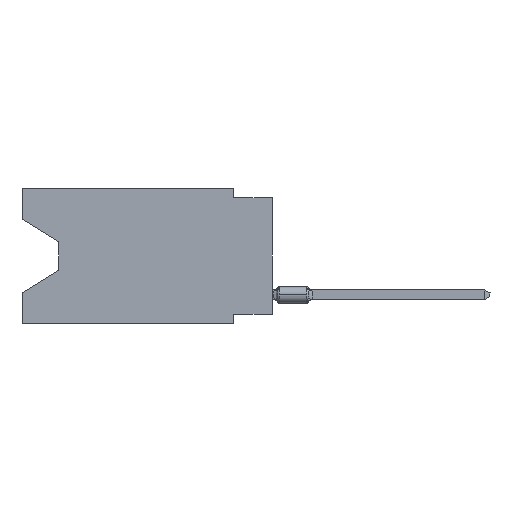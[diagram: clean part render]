
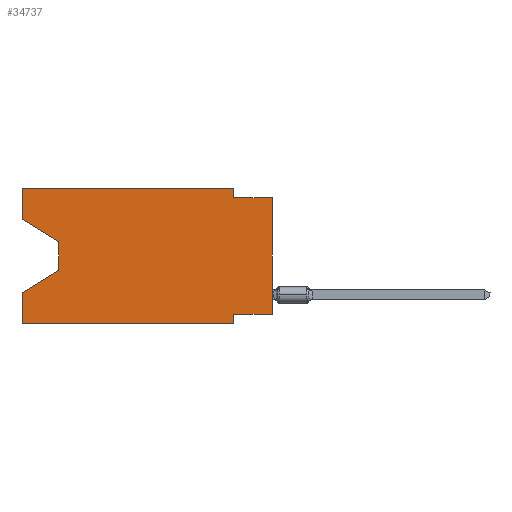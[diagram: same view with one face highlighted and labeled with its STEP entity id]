
A CAD part, left-side view. The second image highlights one B-rep face of the part: STEP entity #34737.
In plain terms, the highlighted planar face has unit normal (-1, 0, 0).
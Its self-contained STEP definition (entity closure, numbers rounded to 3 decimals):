
#1907 = EDGE_CURVE ( 'NONE', #35857, #26477, #60398, .T. ) ;
#2072 = CARTESIAN_POINT ( 'NONE',  ( 0., 16.383, -2.038 ) ) ;
#2202 = VECTOR ( 'NONE', #43808, 1000. ) ;
#2534 = CARTESIAN_POINT ( 'NONE',  ( 0., 2.54, 0. ) ) ;
#2796 = VECTOR ( 'NONE', #10753, 1000. ) ;
#2825 = ORIENTED_EDGE ( 'NONE', *, *, #66326, .F. ) ;
#3435 = DIRECTION ( 'NONE',  ( 0., 0., 1. ) ) ;
#3458 = VECTOR ( 'NONE', #4051, 1000. ) ;
#4051 = DIRECTION ( 'NONE',  ( 0., 1., 0. ) ) ;
#4094 = LINE ( 'NONE', #59790, #44699 ) ;
#4171 = EDGE_CURVE ( 'NONE', #24167, #34870, #17323, .T. ) ;
#4371 = CARTESIAN_POINT ( 'NONE',  ( 0., 0., -8.255 ) ) ;
#5123 = LINE ( 'NONE', #24635, #45087 ) ;
#8419 = EDGE_CURVE ( 'NONE', #58471, #20894, #43483, .T. ) ;
#8764 = CARTESIAN_POINT ( 'NONE',  ( 0., 2.54, 0. ) ) ;
#9741 = CARTESIAN_POINT ( 'NONE',  ( 0., 0., -8.255 ) ) ;
#10753 = DIRECTION ( 'NONE',  ( 0., 0., 1. ) ) ;
#14481 = CARTESIAN_POINT ( 'NONE',  ( 0., 2.54, -0.635 ) ) ;
#14877 = ORIENTED_EDGE ( 'NONE', *, *, #4171, .T. ) ;
#15193 = AXIS2_PLACEMENT_3D ( 'NONE', #42776, #52511, #16956 ) ;
#15799 = CARTESIAN_POINT ( 'NONE',  ( 0., 0., 0. ) ) ;
#16239 = EDGE_LOOP ( 'NONE', ( #27322, #45080, #14877, #50789, #20586, #33544, #38859, #63940, #17327, #30120, #46750, #2825 ) ) ;
#16730 = CARTESIAN_POINT ( 'NONE',  ( 0., 2.54, -8.255 ) ) ;
#16956 = DIRECTION ( 'NONE',  ( 0., 0., -1. ) ) ;
#17323 = LINE ( 'NONE', #44161, #27158 ) ;
#17327 = ORIENTED_EDGE ( 'NONE', *, *, #64099, .F. ) ;
#17516 = LINE ( 'NONE', #24243, #65912 ) ;
#18044 = CARTESIAN_POINT ( 'NONE',  ( 0., 13.97, -5.385 ) ) ;
#19841 = VECTOR ( 'NONE', #53086, 1000. ) ;
#20586 = ORIENTED_EDGE ( 'NONE', *, *, #66115, .T. ) ;
#20894 = VERTEX_POINT ( 'NONE', #2534 ) ;
#21684 = VECTOR ( 'NONE', #27946, 1000. ) ;
#22699 = VERTEX_POINT ( 'NONE', #14481 ) ;
#22721 = VECTOR ( 'NONE', #53522, 1000. ) ;
#22826 = EDGE_CURVE ( 'NONE', #35857, #51320, #30907, .T. ) ;
#23244 = LINE ( 'NONE', #8764, #31380 ) ;
#24167 = VERTEX_POINT ( 'NONE', #18044 ) ;
#24243 = CARTESIAN_POINT ( 'NONE',  ( 0., 0., -0.635 ) ) ;
#24635 = CARTESIAN_POINT ( 'NONE',  ( 0., 2.54, -8.89 ) ) ;
#26477 = VERTEX_POINT ( 'NONE', #16730 ) ;
#27158 = VECTOR ( 'NONE', #63955, 1000. ) ;
#27322 = ORIENTED_EDGE ( 'NONE', *, *, #63907, .T. ) ;
#27339 = CARTESIAN_POINT ( 'NONE',  ( 0., 16.383, -8.89 ) ) ;
#27946 = DIRECTION ( 'NONE',  ( 0., 0., -1. ) ) ;
#29257 = DIRECTION ( 'NONE',  ( 0., 0., -1. ) ) ;
#29989 = DIRECTION ( 'NONE',  ( 0., 0., -1. ) ) ;
#30120 = ORIENTED_EDGE ( 'NONE', *, *, #35765, .F. ) ;
#30907 = LINE ( 'NONE', #15799, #2796 ) ;
#31380 = VECTOR ( 'NONE', #29257, 1000. ) ;
#32416 = CARTESIAN_POINT ( 'NONE',  ( 0., 2.54, -8.89 ) ) ;
#33060 = LINE ( 'NONE', #64259, #22721 ) ;
#33071 = CARTESIAN_POINT ( 'NONE',  ( 0., 16.383, 0. ) ) ;
#33544 = ORIENTED_EDGE ( 'NONE', *, *, #40158, .F. ) ;
#34280 = CARTESIAN_POINT ( 'NONE',  ( 0., 16.383, -2.038 ) ) ;
#34737 = ADVANCED_FACE ( 'NONE', ( #48480 ), #47822, .F. ) ;
#34870 = VERTEX_POINT ( 'NONE', #40060 ) ;
#35096 = CARTESIAN_POINT ( 'NONE',  ( 0., 0., -0.635 ) ) ;
#35765 = EDGE_CURVE ( 'NONE', #20894, #22699, #23244, .T. ) ;
#35857 = VERTEX_POINT ( 'NONE', #9741 ) ;
#38859 = ORIENTED_EDGE ( 'NONE', *, *, #1907, .F. ) ;
#40060 = CARTESIAN_POINT ( 'NONE',  ( 0., 16.383, -6.852 ) ) ;
#40158 = EDGE_CURVE ( 'NONE', #26477, #41803, #5123, .T. ) ;
#40471 = LINE ( 'NONE', #45521, #54323 ) ;
#41803 = VERTEX_POINT ( 'NONE', #32416 ) ;
#41937 = EDGE_CURVE ( 'NONE', #49698, #34870, #33060, .T. ) ;
#42776 = CARTESIAN_POINT ( 'NONE',  ( 0., 16.383, 0. ) ) ;
#43483 = LINE ( 'NONE', #33071, #2202 ) ;
#43808 = DIRECTION ( 'NONE',  ( 0., -1., 0. ) ) ;
#44161 = CARTESIAN_POINT ( 'NONE',  ( 0., 13.97, -5.385 ) ) ;
#44683 = DIRECTION ( 'NONE',  ( 0., -1., 0. ) ) ;
#44699 = VECTOR ( 'NONE', #3435, 1000. ) ;
#45080 = ORIENTED_EDGE ( 'NONE', *, *, #54404, .T. ) ;
#45087 = VECTOR ( 'NONE', #29989, 1000. ) ;
#45521 = CARTESIAN_POINT ( 'NONE',  ( 0., 16.383, -8.89 ) ) ;
#45600 = VERTEX_POINT ( 'NONE', #56884 ) ;
#46750 = ORIENTED_EDGE ( 'NONE', *, *, #8419, .F. ) ;
#47822 = PLANE ( 'NONE',  #15193 ) ;
#48480 = FACE_OUTER_BOUND ( 'NONE', #16239, .T. ) ;
#49698 = VERTEX_POINT ( 'NONE', #27339 ) ;
#50789 = ORIENTED_EDGE ( 'NONE', *, *, #41937, .F. ) ;
#51320 = VERTEX_POINT ( 'NONE', #35096 ) ;
#52511 = DIRECTION ( 'NONE',  ( 1., 0., 0. ) ) ;
#52977 = CARTESIAN_POINT ( 'NONE',  ( 0., 16.383, 0. ) ) ;
#53086 = DIRECTION ( 'NONE',  ( 0., -0.855, -0.519 ) ) ;
#53419 = CARTESIAN_POINT ( 'NONE',  ( 0., 13.97, -3.505 ) ) ;
#53522 = DIRECTION ( 'NONE',  ( 0., 0., 1. ) ) ;
#54323 = VECTOR ( 'NONE', #54920, 1000. ) ;
#54404 = EDGE_CURVE ( 'NONE', #45600, #24167, #63828, .T. ) ;
#54920 = DIRECTION ( 'NONE',  ( 0., -1., 0. ) ) ;
#56884 = CARTESIAN_POINT ( 'NONE',  ( 0., 13.97, -3.505 ) ) ;
#57118 = LINE ( 'NONE', #2072, #19841 ) ;
#58471 = VERTEX_POINT ( 'NONE', #52977 ) ;
#59790 = CARTESIAN_POINT ( 'NONE',  ( 0., 16.383, 0. ) ) ;
#60398 = LINE ( 'NONE', #4371, #3458 ) ;
#63828 = LINE ( 'NONE', #53419, #21684 ) ;
#63907 = EDGE_CURVE ( 'NONE', #64030, #45600, #57118, .T. ) ;
#63940 = ORIENTED_EDGE ( 'NONE', *, *, #22826, .T. ) ;
#63955 = DIRECTION ( 'NONE',  ( 0., 0.855, -0.519 ) ) ;
#64030 = VERTEX_POINT ( 'NONE', #34280 ) ;
#64099 = EDGE_CURVE ( 'NONE', #22699, #51320, #17516, .T. ) ;
#64259 = CARTESIAN_POINT ( 'NONE',  ( 0., 16.383, 0. ) ) ;
#65912 = VECTOR ( 'NONE', #44683, 1000. ) ;
#66115 = EDGE_CURVE ( 'NONE', #49698, #41803, #40471, .T. ) ;
#66326 = EDGE_CURVE ( 'NONE', #64030, #58471, #4094, .T. ) ;
